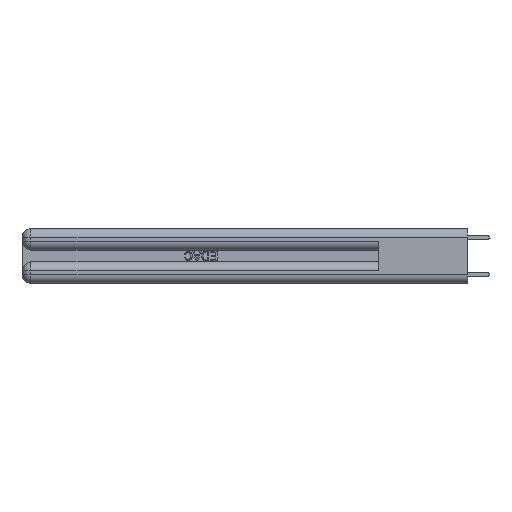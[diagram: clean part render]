
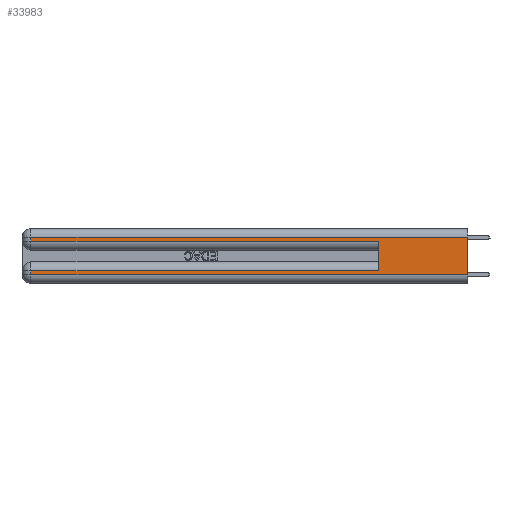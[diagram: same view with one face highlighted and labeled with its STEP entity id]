
A CAD part, left-side view. The second image highlights one B-rep face of the part: STEP entity #33983.
In plain terms, the highlighted planar face has unit normal (-1, 0, 0).
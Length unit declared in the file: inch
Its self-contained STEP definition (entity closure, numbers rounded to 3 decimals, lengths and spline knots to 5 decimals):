
#78 = VERTEX_POINT ( 'NONE', #13115 ) ;
#403 = CARTESIAN_POINT ( 'NONE',  ( 0., 0., 0.31 ) ) ;
#923 = VERTEX_POINT ( 'NONE', #21509 ) ;
#1407 = EDGE_LOOP ( 'NONE', ( #32284, #11805, #2708, #34666, #25112, #34316, #12381, #20301 ) ) ;
#2202 = DIRECTION ( 'NONE',  ( 0., 0., -1. ) ) ;
#2708 = ORIENTED_EDGE ( 'NONE', *, *, #4843, .T. ) ;
#3611 = CARTESIAN_POINT ( 'NONE',  ( 0., 2.94, 0.37 ) ) ;
#3896 = EDGE_CURVE ( 'NONE', #923, #34337, #12949, .T. ) ;
#4820 = CARTESIAN_POINT ( 'NONE',  ( 0., 0., 0.37 ) ) ;
#4843 = EDGE_CURVE ( 'NONE', #22232, #923, #31430, .T. ) ;
#4928 = PLANE ( 'NONE',  #7739 ) ;
#5468 = LINE ( 'NONE', #9136, #27462 ) ;
#5483 = EDGE_CURVE ( 'NONE', #15676, #78, #5468, .T. ) ;
#6934 = DIRECTION ( 'NONE',  ( 0., -1., 0. ) ) ;
#7442 = DIRECTION ( 'NONE',  ( 0., 0., -1. ) ) ;
#7739 = AXIS2_PLACEMENT_3D ( 'NONE', #4820, #10353, #7442 ) ;
#8625 = LINE ( 'NONE', #14432, #9092 ) ;
#8890 = CARTESIAN_POINT ( 'NONE',  ( 0., 0.6, 0.285 ) ) ;
#8973 = VECTOR ( 'NONE', #11937, 39.37008 ) ;
#9092 = VECTOR ( 'NONE', #17307, 39.37008 ) ;
#9136 = CARTESIAN_POINT ( 'NONE',  ( 0., 0., 0.06 ) ) ;
#9308 = CARTESIAN_POINT ( 'NONE',  ( 0., 0., 0.285 ) ) ;
#9746 = VERTEX_POINT ( 'NONE', #403 ) ;
#10330 = LINE ( 'NONE', #24394, #34548 ) ;
#10353 = DIRECTION ( 'NONE',  ( 1., 0., 0. ) ) ;
#10516 = EDGE_CURVE ( 'NONE', #21696, #34337, #8625, .T. ) ;
#11805 = ORIENTED_EDGE ( 'NONE', *, *, #34445, .T. ) ;
#11937 = DIRECTION ( 'NONE',  ( 0., 0., -1. ) ) ;
#12381 = ORIENTED_EDGE ( 'NONE', *, *, #34697, .T. ) ;
#12949 = LINE ( 'NONE', #9308, #12965 ) ;
#12965 = VECTOR ( 'NONE', #23291, 39.37008 ) ;
#13115 = CARTESIAN_POINT ( 'NONE',  ( 0., 0., 0.06 ) ) ;
#13638 = LINE ( 'NONE', #23100, #25715 ) ;
#13728 = VERTEX_POINT ( 'NONE', #28769 ) ;
#13837 = CARTESIAN_POINT ( 'NONE',  ( 0., 2.94, 0.31 ) ) ;
#13848 = FACE_OUTER_BOUND ( 'NONE', #1407, .T. ) ;
#14005 = CARTESIAN_POINT ( 'NONE',  ( 0., 2.94, 0.06 ) ) ;
#14432 = CARTESIAN_POINT ( 'NONE',  ( 0., 0.6, 0.145 ) ) ;
#15676 = VERTEX_POINT ( 'NONE', #14005 ) ;
#15944 = CARTESIAN_POINT ( 'NONE',  ( 0., 0.6, 0.085 ) ) ;
#16567 = EDGE_CURVE ( 'NONE', #9746, #78, #13638, .T. ) ;
#17307 = DIRECTION ( 'NONE',  ( 0., 0., 1. ) ) ;
#19031 = VECTOR ( 'NONE', #34359, 39.37008 ) ;
#20301 = ORIENTED_EDGE ( 'NONE', *, *, #5483, .T. ) ;
#21509 = CARTESIAN_POINT ( 'NONE',  ( 0., 2.94, 0.285 ) ) ;
#21696 = VERTEX_POINT ( 'NONE', #15944 ) ;
#22232 = VERTEX_POINT ( 'NONE', #13837 ) ;
#22923 = LINE ( 'NONE', #26353, #19031 ) ;
#23100 = CARTESIAN_POINT ( 'NONE',  ( 0., 0., 0.37 ) ) ;
#23291 = DIRECTION ( 'NONE',  ( 0., -1., 0. ) ) ;
#23317 = LINE ( 'NONE', #31541, #29348 ) ;
#23354 = DIRECTION ( 'NONE',  ( 0., 1., 0. ) ) ;
#24394 = CARTESIAN_POINT ( 'NONE',  ( 0., 2.94, 0.37 ) ) ;
#25112 = ORIENTED_EDGE ( 'NONE', *, *, #10516, .F. ) ;
#25715 = VECTOR ( 'NONE', #32491, 39.37008 ) ;
#26353 = CARTESIAN_POINT ( 'NONE',  ( 0., 0., 0.085 ) ) ;
#27462 = VECTOR ( 'NONE', #6934, 39.37008 ) ;
#27668 = EDGE_CURVE ( 'NONE', #21696, #13728, #22923, .T. ) ;
#28769 = CARTESIAN_POINT ( 'NONE',  ( 0., 2.94, 0.085 ) ) ;
#29348 = VECTOR ( 'NONE', #23354, 39.37008 ) ;
#31430 = LINE ( 'NONE', #3611, #8973 ) ;
#31541 = CARTESIAN_POINT ( 'NONE',  ( 0., 0., 0.31 ) ) ;
#32284 = ORIENTED_EDGE ( 'NONE', *, *, #16567, .F. ) ;
#32491 = DIRECTION ( 'NONE',  ( 0., 0., -1. ) ) ;
#33983 = ADVANCED_FACE ( 'NONE', ( #13848 ), #4928, .F. ) ;
#34316 = ORIENTED_EDGE ( 'NONE', *, *, #27668, .T. ) ;
#34337 = VERTEX_POINT ( 'NONE', #8890 ) ;
#34359 = DIRECTION ( 'NONE',  ( 0., 1., 0. ) ) ;
#34445 = EDGE_CURVE ( 'NONE', #9746, #22232, #23317, .T. ) ;
#34548 = VECTOR ( 'NONE', #2202, 39.37008 ) ;
#34666 = ORIENTED_EDGE ( 'NONE', *, *, #3896, .T. ) ;
#34697 = EDGE_CURVE ( 'NONE', #13728, #15676, #10330, .T. ) ;
